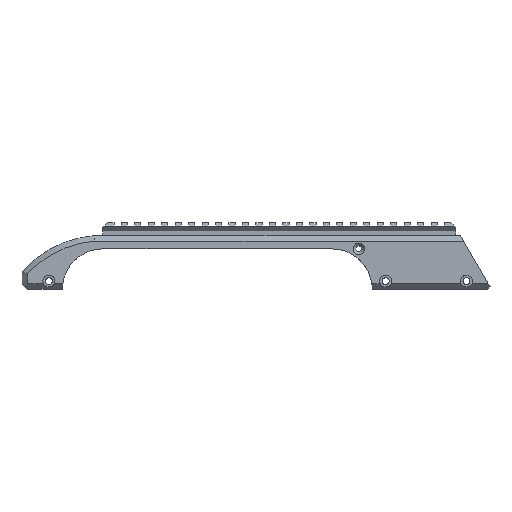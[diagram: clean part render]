
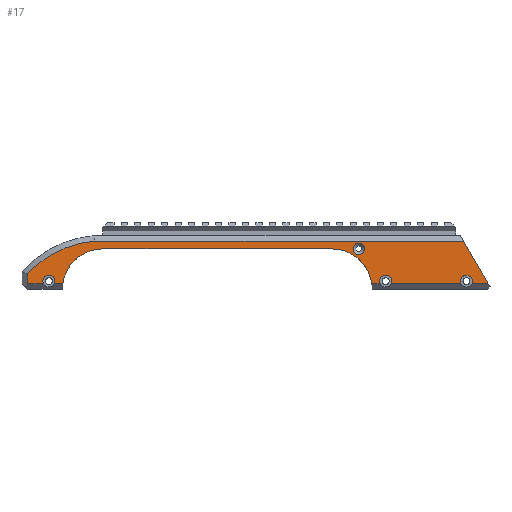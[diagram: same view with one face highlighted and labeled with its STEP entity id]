
A CAD part, left-side view. The second image highlights one B-rep face of the part: STEP entity #17.
In plain terms, the highlighted planar face has unit normal (-1, 0, 0).
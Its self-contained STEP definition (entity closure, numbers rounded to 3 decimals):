
#17 = ADVANCED_FACE('',(#18,#154),#165,.F.);
#18 = FACE_BOUND('',#19,.F.);
#19 = EDGE_LOOP('',(#20,#30,#38,#46,#54,#63,#71,#80,#88,#97,#105,#114,
    #122,#131,#139,#147));
#20 = ORIENTED_EDGE('',*,*,#21,.F.);
#21 = EDGE_CURVE('',#22,#24,#26,.T.);
#22 = VERTEX_POINT('',#23);
#23 = CARTESIAN_POINT('',(-15.,-152.808,15.757));
#24 = VERTEX_POINT('',#25);
#25 = CARTESIAN_POINT('',(-15.,121.068,15.757));
#26 = LINE('',#27,#28);
#27 = CARTESIAN_POINT('',(-15.,-175.,15.757));
#28 = VECTOR('',#29,1.);
#29 = DIRECTION('',(0.,1.,0.));
#30 = ORIENTED_EDGE('',*,*,#31,.F.);
#31 = EDGE_CURVE('',#32,#22,#34,.T.);
#32 = VERTEX_POINT('',#33);
#33 = CARTESIAN_POINT('',(-15.,-170.757,-15.331));
#34 = LINE('',#35,#36);
#35 = CARTESIAN_POINT('',(-15.,-187.679,-44.641));
#36 = VECTOR('',#37,1.);
#37 = DIRECTION('',(0.,0.5,0.866));
#38 = ORIENTED_EDGE('',*,*,#39,.F.);
#39 = EDGE_CURVE('',#40,#32,#42,.T.);
#40 = VERTEX_POINT('',#41);
#41 = CARTESIAN_POINT('',(-15.,-170.757,-15.757));
#42 = LINE('',#43,#44);
#43 = CARTESIAN_POINT('',(-15.,-170.757,-20.));
#44 = VECTOR('',#45,1.);
#45 = DIRECTION('',(0.,0.,1.));
#46 = ORIENTED_EDGE('',*,*,#47,.T.);
#47 = EDGE_CURVE('',#40,#48,#50,.T.);
#48 = VERTEX_POINT('',#49);
#49 = CARTESIAN_POINT('',(-15.,-159.143,-15.757));
#50 = LINE('',#51,#52);
#51 = CARTESIAN_POINT('',(-15.,-175.,-15.757));
#52 = VECTOR('',#53,1.);
#53 = DIRECTION('',(0.,1.,0.));
#54 = ORIENTED_EDGE('',*,*,#55,.F.);
#55 = EDGE_CURVE('',#56,#48,#58,.T.);
#56 = VERTEX_POINT('',#57);
#57 = CARTESIAN_POINT('',(-15.,-150.857,-15.757));
#58 = CIRCLE('',#59,4.5);
#59 = AXIS2_PLACEMENT_3D('',#60,#61,#62);
#60 = CARTESIAN_POINT('',(-15.,-155.,-14.));
#61 = DIRECTION('',(1.,-0.,0.));
#62 = DIRECTION('',(0.,0.,-1.));
#63 = ORIENTED_EDGE('',*,*,#64,.T.);
#64 = EDGE_CURVE('',#56,#65,#67,.T.);
#65 = VERTEX_POINT('',#66);
#66 = CARTESIAN_POINT('',(-15.,-99.143,-15.757));
#67 = LINE('',#68,#69);
#68 = CARTESIAN_POINT('',(-15.,-175.,-15.757));
#69 = VECTOR('',#70,1.);
#70 = DIRECTION('',(0.,1.,0.));
#71 = ORIENTED_EDGE('',*,*,#72,.F.);
#72 = EDGE_CURVE('',#73,#65,#75,.T.);
#73 = VERTEX_POINT('',#74);
#74 = CARTESIAN_POINT('',(-15.,-90.857,-15.757));
#75 = CIRCLE('',#76,4.5);
#76 = AXIS2_PLACEMENT_3D('',#77,#78,#79);
#77 = CARTESIAN_POINT('',(-15.,-95.,-14.));
#78 = DIRECTION('',(1.,-0.,0.));
#79 = DIRECTION('',(0.,0.,-1.));
#80 = ORIENTED_EDGE('',*,*,#81,.T.);
#81 = EDGE_CURVE('',#73,#82,#84,.T.);
#82 = VERTEX_POINT('',#83);
#83 = CARTESIAN_POINT('',(-15.,-84.698,-15.757));
#84 = LINE('',#85,#86);
#85 = CARTESIAN_POINT('',(-15.,-175.,-15.757));
#86 = VECTOR('',#87,1.);
#87 = DIRECTION('',(0.,1.,0.));
#88 = ORIENTED_EDGE('',*,*,#89,.T.);
#89 = EDGE_CURVE('',#82,#90,#92,.T.);
#90 = VERTEX_POINT('',#91);
#91 = CARTESIAN_POINT('',(-15.,-55.,10.));
#92 = CIRCLE('',#93,30.);
#93 = AXIS2_PLACEMENT_3D('',#94,#95,#96);
#94 = CARTESIAN_POINT('',(-15.,-55.,-20.));
#95 = DIRECTION('',(-1.,-0.,0.));
#96 = DIRECTION('',(0.,0.,-1.));
#97 = ORIENTED_EDGE('',*,*,#98,.T.);
#98 = EDGE_CURVE('',#90,#99,#101,.T.);
#99 = VERTEX_POINT('',#100);
#100 = CARTESIAN_POINT('',(-15.,115.,10.));
#101 = LINE('',#102,#103);
#102 = CARTESIAN_POINT('',(-15.,-115.,10.));
#103 = VECTOR('',#104,1.);
#104 = DIRECTION('',(-0.,1.,0.));
#105 = ORIENTED_EDGE('',*,*,#106,.T.);
#106 = EDGE_CURVE('',#99,#107,#109,.T.);
#107 = VERTEX_POINT('',#108);
#108 = CARTESIAN_POINT('',(-15.,144.698,-15.757));
#109 = CIRCLE('',#110,30.);
#110 = AXIS2_PLACEMENT_3D('',#111,#112,#113);
#111 = CARTESIAN_POINT('',(-15.,115.,-20.));
#112 = DIRECTION('',(-1.,-0.,0.));
#113 = DIRECTION('',(0.,0.,-1.));
#114 = ORIENTED_EDGE('',*,*,#115,.T.);
#115 = EDGE_CURVE('',#107,#116,#118,.T.);
#116 = VERTEX_POINT('',#117);
#117 = CARTESIAN_POINT('',(-15.,150.857,-15.757));
#118 = LINE('',#119,#120);
#119 = CARTESIAN_POINT('',(-15.,-175.,-15.757));
#120 = VECTOR('',#121,1.);
#121 = DIRECTION('',(0.,1.,0.));
#122 = ORIENTED_EDGE('',*,*,#123,.F.);
#123 = EDGE_CURVE('',#124,#116,#126,.T.);
#124 = VERTEX_POINT('',#125);
#125 = CARTESIAN_POINT('',(-15.,159.143,-15.757));
#126 = CIRCLE('',#127,4.5);
#127 = AXIS2_PLACEMENT_3D('',#128,#129,#130);
#128 = CARTESIAN_POINT('',(-15.,155.,-14.));
#129 = DIRECTION('',(1.,-0.,0.));
#130 = DIRECTION('',(0.,0.,-1.));
#131 = ORIENTED_EDGE('',*,*,#132,.T.);
#132 = EDGE_CURVE('',#124,#133,#135,.T.);
#133 = VERTEX_POINT('',#134);
#134 = CARTESIAN_POINT('',(-15.,170.757,-15.757));
#135 = LINE('',#136,#137);
#136 = CARTESIAN_POINT('',(-15.,-175.,-15.757));
#137 = VECTOR('',#138,1.);
#138 = DIRECTION('',(0.,1.,0.));
#139 = ORIENTED_EDGE('',*,*,#140,.T.);
#140 = EDGE_CURVE('',#133,#141,#143,.T.);
#141 = VERTEX_POINT('',#142);
#142 = CARTESIAN_POINT('',(-15.,170.757,-8.356));
#143 = LINE('',#144,#145);
#144 = CARTESIAN_POINT('',(-15.,170.757,-20.));
#145 = VECTOR('',#146,1.);
#146 = DIRECTION('',(0.,0.,1.));
#147 = ORIENTED_EDGE('',*,*,#148,.T.);
#148 = EDGE_CURVE('',#141,#24,#149,.T.);
#149 = CIRCLE('',#150,76.);
#150 = AXIS2_PLACEMENT_3D('',#151,#152,#153);
#151 = CARTESIAN_POINT('',(-15.,115.,-60.));
#152 = DIRECTION('',(1.,-0.,0.));
#153 = DIRECTION('',(0.,0.,-1.));
#154 = FACE_BOUND('',#155,.F.);
#155 = EDGE_LOOP('',(#156));
#156 = ORIENTED_EDGE('',*,*,#157,.T.);
#157 = EDGE_CURVE('',#158,#158,#160,.T.);
#158 = VERTEX_POINT('',#159);
#159 = CARTESIAN_POINT('',(-15.,-75.,14.2));
#160 = CIRCLE('',#161,4.2);
#161 = AXIS2_PLACEMENT_3D('',#162,#163,#164);
#162 = CARTESIAN_POINT('',(-15.,-75.,10.));
#163 = DIRECTION('',(-1.,0.,0.));
#164 = DIRECTION('',(0.,0.,1.));
#165 = PLANE('',#166);
#166 = AXIS2_PLACEMENT_3D('',#167,#168,#169);
#167 = CARTESIAN_POINT('',(-15.,-175.,-20.));
#168 = DIRECTION('',(1.,0.,0.));
#169 = DIRECTION('',(0.,0.,1.));
